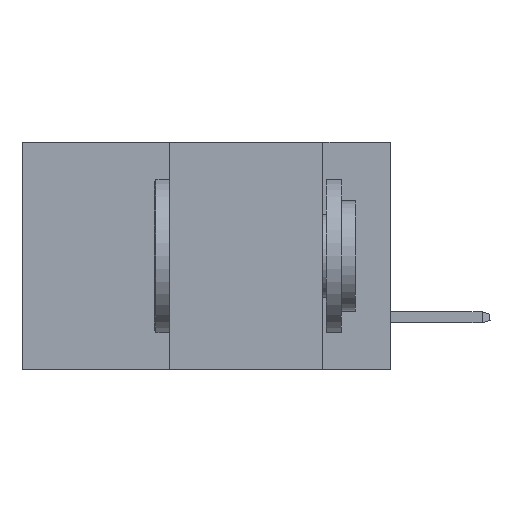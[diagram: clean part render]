
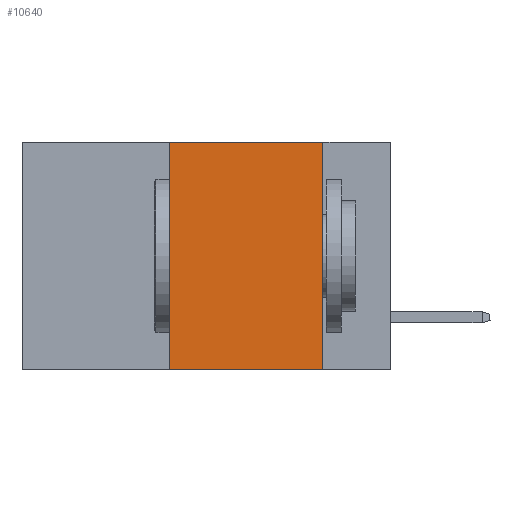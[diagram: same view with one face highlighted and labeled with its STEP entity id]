
A CAD part, left-side view. The second image highlights one B-rep face of the part: STEP entity #10640.
In plain terms, the highlighted planar face has unit normal (-1, 0, 0).
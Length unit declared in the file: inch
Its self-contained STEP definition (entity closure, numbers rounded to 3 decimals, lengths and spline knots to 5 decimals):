
#169 = VECTOR ( 'NONE', #16595, 39.37008 ) ;
#3023 = EDGE_CURVE ( 'NONE', #36720, #29989, #18023, .T. ) ;
#4191 = CARTESIAN_POINT ( 'NONE',  ( 0., 0.11, 0. ) ) ;
#4229 = CARTESIAN_POINT ( 'NONE',  ( 0., 0.6, 0. ) ) ;
#5129 = CARTESIAN_POINT ( 'NONE',  ( 0., 0.36, 0. ) ) ;
#5339 = ORIENTED_EDGE ( 'NONE', *, *, #13594, .F. ) ;
#6480 = AXIS2_PLACEMENT_3D ( 'NONE', #4229, #9515, #34930 ) ;
#6977 = VECTOR ( 'NONE', #37667, 39.37008 ) ;
#7561 = VERTEX_POINT ( 'NONE', #5129 ) ;
#8049 = DIRECTION ( 'NONE',  ( 0., -1., 0. ) ) ;
#9440 = EDGE_CURVE ( 'NONE', #9542, #7561, #15148, .T. ) ;
#9515 = DIRECTION ( 'NONE',  ( 1., 0., 0. ) ) ;
#9542 = VERTEX_POINT ( 'NONE', #24319 ) ;
#10640 = ADVANCED_FACE ( 'NONE', ( #32830 ), #25672, .F. ) ;
#11725 = VECTOR ( 'NONE', #8049, 39.37008 ) ;
#13594 = EDGE_CURVE ( 'NONE', #7561, #36720, #32585, .T. ) ;
#15005 = DIRECTION ( 'NONE',  ( 0., 0., 1. ) ) ;
#15148 = LINE ( 'NONE', #33437, #31939 ) ;
#16595 = DIRECTION ( 'NONE',  ( 0., 0., -1. ) ) ;
#17582 = CARTESIAN_POINT ( 'NONE',  ( 0., 0.6, -0.37 ) ) ;
#17805 = ORIENTED_EDGE ( 'NONE', *, *, #9440, .F. ) ;
#18023 = LINE ( 'NONE', #4191, #169 ) ;
#18817 = CARTESIAN_POINT ( 'NONE',  ( 0., 0.11, -0.37 ) ) ;
#19893 = LINE ( 'NONE', #17582, #11725 ) ;
#20111 = ORIENTED_EDGE ( 'NONE', *, *, #33398, .T. ) ;
#22734 = EDGE_LOOP ( 'NONE', ( #35575, #5339, #17805, #20111 ) ) ;
#24319 = CARTESIAN_POINT ( 'NONE',  ( 0., 0.36, -0.37 ) ) ;
#25672 = PLANE ( 'NONE',  #6480 ) ;
#28317 = CARTESIAN_POINT ( 'NONE',  ( 0., 0.6, 0. ) ) ;
#29989 = VERTEX_POINT ( 'NONE', #18817 ) ;
#31939 = VECTOR ( 'NONE', #15005, 39.37008 ) ;
#32585 = LINE ( 'NONE', #28317, #6977 ) ;
#32830 = FACE_OUTER_BOUND ( 'NONE', #22734, .T. ) ;
#33398 = EDGE_CURVE ( 'NONE', #9542, #29989, #19893, .T. ) ;
#33437 = CARTESIAN_POINT ( 'NONE',  ( 0., 0.36, 0. ) ) ;
#33695 = CARTESIAN_POINT ( 'NONE',  ( 0., 0.11, 0. ) ) ;
#34930 = DIRECTION ( 'NONE',  ( 0., 0., -1. ) ) ;
#35575 = ORIENTED_EDGE ( 'NONE', *, *, #3023, .F. ) ;
#36720 = VERTEX_POINT ( 'NONE', #33695 ) ;
#37667 = DIRECTION ( 'NONE',  ( 0., -1., 0. ) ) ;
